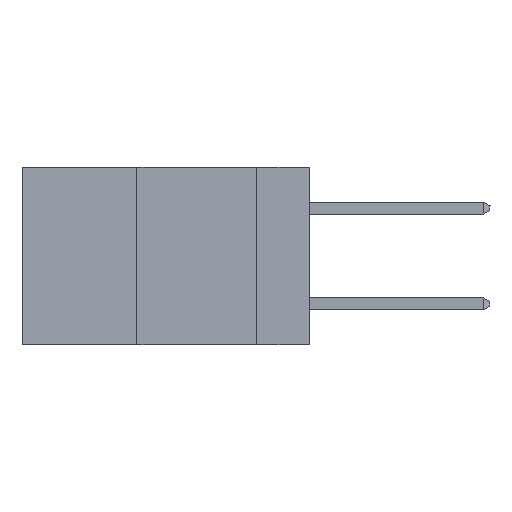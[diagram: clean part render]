
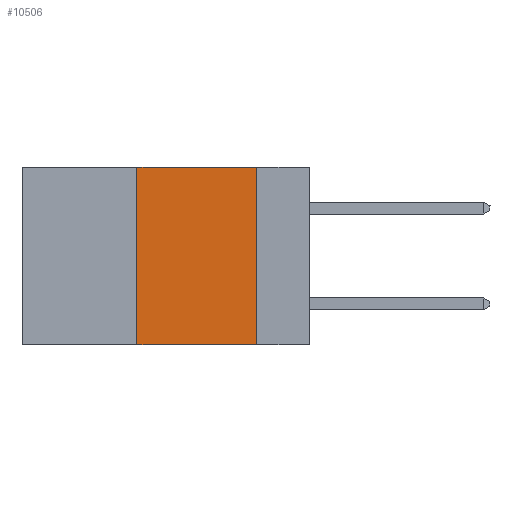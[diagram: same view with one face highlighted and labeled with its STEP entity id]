
A CAD part, left-side view. The second image highlights one B-rep face of the part: STEP entity #10506.
In plain terms, the highlighted planar face has unit normal (-1, 0, 0).
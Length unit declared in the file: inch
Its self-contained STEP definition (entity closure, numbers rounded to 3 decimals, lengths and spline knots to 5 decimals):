
#979 = EDGE_CURVE ( 'NONE', #30153, #25887, #9330, .T. ) ;
#2397 = EDGE_CURVE ( 'NONE', #25887, #43336, #17100, .T. ) ;
#3181 = VECTOR ( 'NONE', #4820, 39.37008 ) ;
#3444 = LINE ( 'NONE', #8576, #3181 ) ;
#4820 = DIRECTION ( 'NONE',  ( 0., 0., -1. ) ) ;
#7867 = EDGE_LOOP ( 'NONE', ( #8630, #9409, #10061, #11073 ) ) ;
#8576 = CARTESIAN_POINT ( 'NONE',  ( 0., 0.11, 0. ) ) ;
#8630 = ORIENTED_EDGE ( 'NONE', *, *, #13042, .F. ) ;
#9330 = LINE ( 'NONE', #11415, #9656 ) ;
#9409 = ORIENTED_EDGE ( 'NONE', *, *, #2397, .F. ) ;
#9478 = VECTOR ( 'NONE', #18620, 39.37008 ) ;
#9656 = VECTOR ( 'NONE', #35798, 39.37008 ) ;
#10061 = ORIENTED_EDGE ( 'NONE', *, *, #979, .F. ) ;
#10506 = ADVANCED_FACE ( 'NONE', ( #23264 ), #11746, .F. ) ;
#11073 = ORIENTED_EDGE ( 'NONE', *, *, #35201, .T. ) ;
#11415 = CARTESIAN_POINT ( 'NONE',  ( 0., 0.36, 0. ) ) ;
#11746 = PLANE ( 'NONE',  #17536 ) ;
#13042 = EDGE_CURVE ( 'NONE', #43336, #29706, #3444, .T. ) ;
#14738 = CARTESIAN_POINT ( 'NONE',  ( 0., 0.6, 0. ) ) ;
#17100 = LINE ( 'NONE', #14738, #18128 ) ;
#17536 = AXIS2_PLACEMENT_3D ( 'NONE', #36111, #18987, #42687 ) ;
#18128 = VECTOR ( 'NONE', #18363, 39.37008 ) ;
#18363 = DIRECTION ( 'NONE',  ( 0., -1., 0. ) ) ;
#18620 = DIRECTION ( 'NONE',  ( 0., -1., 0. ) ) ;
#18987 = DIRECTION ( 'NONE',  ( 1., 0., 0. ) ) ;
#23264 = FACE_OUTER_BOUND ( 'NONE', #7867, .T. ) ;
#25887 = VERTEX_POINT ( 'NONE', #33993 ) ;
#27355 = LINE ( 'NONE', #39070, #9478 ) ;
#29420 = CARTESIAN_POINT ( 'NONE',  ( 0., 0.11, -0.37 ) ) ;
#29706 = VERTEX_POINT ( 'NONE', #29420 ) ;
#30153 = VERTEX_POINT ( 'NONE', #44700 ) ;
#33993 = CARTESIAN_POINT ( 'NONE',  ( 0., 0.36, 0. ) ) ;
#35201 = EDGE_CURVE ( 'NONE', #30153, #29706, #27355, .T. ) ;
#35798 = DIRECTION ( 'NONE',  ( 0., 0., 1. ) ) ;
#36111 = CARTESIAN_POINT ( 'NONE',  ( 0., 0.6, 0. ) ) ;
#39070 = CARTESIAN_POINT ( 'NONE',  ( 0., 0.6, -0.37 ) ) ;
#39921 = CARTESIAN_POINT ( 'NONE',  ( 0., 0.11, 0. ) ) ;
#42687 = DIRECTION ( 'NONE',  ( 0., 0., -1. ) ) ;
#43336 = VERTEX_POINT ( 'NONE', #39921 ) ;
#44700 = CARTESIAN_POINT ( 'NONE',  ( 0., 0.36, -0.37 ) ) ;
